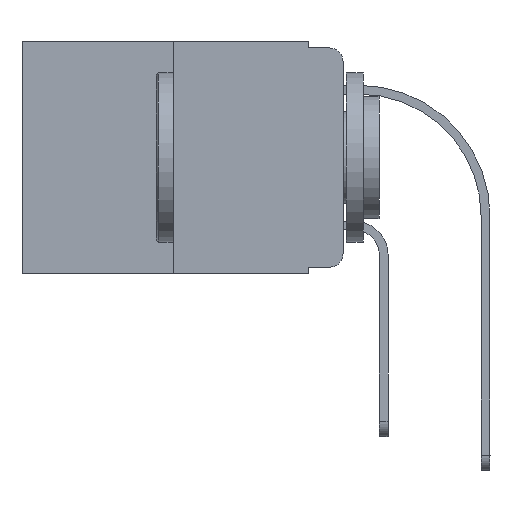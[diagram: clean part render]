
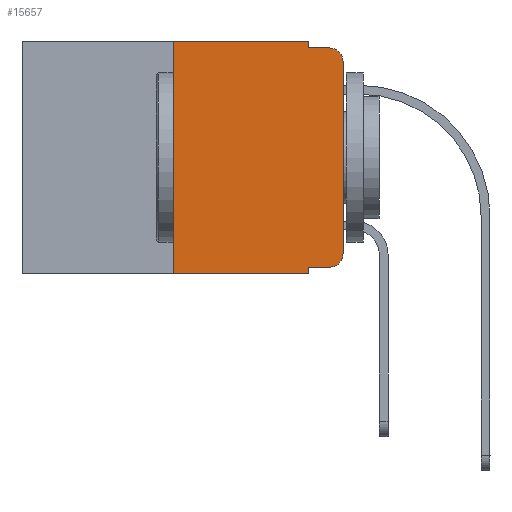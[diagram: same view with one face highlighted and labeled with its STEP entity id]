
A CAD part, left-side view. The second image highlights one B-rep face of the part: STEP entity #15657.
In plain terms, the highlighted planar face has unit normal (-1, 0, 0).
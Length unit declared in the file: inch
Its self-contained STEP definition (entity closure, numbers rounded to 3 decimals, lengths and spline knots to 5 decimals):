
#469 = VECTOR ( 'NONE', #5911, 39.37008 ) ;
#667 = EDGE_CURVE ( 'NONE', #11719, #19846, #1559, .T. ) ;
#905 = AXIS2_PLACEMENT_3D ( 'NONE', #5419, #11566, #17721 ) ;
#948 = CARTESIAN_POINT ( 'NONE',  ( 0., 0.051, 0. ) ) ;
#1408 = LINE ( 'NONE', #10692, #19639 ) ;
#1559 = LINE ( 'NONE', #7807, #7403 ) ;
#1925 = VERTEX_POINT ( 'NONE', #3932 ) ;
#1961 = LINE ( 'NONE', #11256, #14362 ) ;
#2019 = ORIENTED_EDGE ( 'NONE', *, *, #12223, .T. ) ;
#2073 = DIRECTION ( 'NONE',  ( 1., 0., 0. ) ) ;
#2264 = CARTESIAN_POINT ( 'NONE',  ( 0., 0.25, 0. ) ) ;
#2600 = CARTESIAN_POINT ( 'NONE',  ( 0., 0.051, 0. ) ) ;
#3450 = ORIENTED_EDGE ( 'NONE', *, *, #13535, .T. ) ;
#3794 = DIRECTION ( 'NONE',  ( 0., 0., -1. ) ) ;
#3808 = VERTEX_POINT ( 'NONE', #15187 ) ;
#3932 = CARTESIAN_POINT ( 'NONE',  ( 0., 0.051, -0.01 ) ) ;
#4041 = EDGE_CURVE ( 'NONE', #3808, #6773, #12874, .T. ) ;
#4103 = ORIENTED_EDGE ( 'NONE', *, *, #8879, .T. ) ;
#4409 = ORIENTED_EDGE ( 'NONE', *, *, #13688, .F. ) ;
#4512 = VECTOR ( 'NONE', #7450, 39.37008 ) ;
#4573 = ORIENTED_EDGE ( 'NONE', *, *, #9491, .F. ) ;
#4857 = CARTESIAN_POINT ( 'NONE',  ( 0., 0.02, -0.333 ) ) ;
#5004 = DIRECTION ( 'NONE',  ( 0., 0., 1. ) ) ;
#5223 = CARTESIAN_POINT ( 'NONE',  ( 0., 0.473, 0. ) ) ;
#5419 = CARTESIAN_POINT ( 'NONE',  ( 0., 0.02, -0.313 ) ) ;
#5911 = DIRECTION ( 'NONE',  ( 0., 0., -1. ) ) ;
#6040 = CARTESIAN_POINT ( 'NONE',  ( 0., 0.25, 0. ) ) ;
#6282 = CARTESIAN_POINT ( 'NONE',  ( 0., 0.25, -0.343 ) ) ;
#6498 = ORIENTED_EDGE ( 'NONE', *, *, #667, .T. ) ;
#6768 = CARTESIAN_POINT ( 'NONE',  ( 0., 0.02, -0.03 ) ) ;
#6773 = VERTEX_POINT ( 'NONE', #13117 ) ;
#7403 = VECTOR ( 'NONE', #5004, 39.37008 ) ;
#7450 = DIRECTION ( 'NONE',  ( 0., 0., 1. ) ) ;
#7468 = VERTEX_POINT ( 'NONE', #2264 ) ;
#7784 = DIRECTION ( 'NONE',  ( 0., -1., 0. ) ) ;
#7807 = CARTESIAN_POINT ( 'NONE',  ( 0., 0., 0. ) ) ;
#8496 = AXIS2_PLACEMENT_3D ( 'NONE', #5223, #2073, #19440 ) ;
#8706 = ORIENTED_EDGE ( 'NONE', *, *, #9300, .F. ) ;
#8800 = CARTESIAN_POINT ( 'NONE',  ( 0., 0.473, -0.343 ) ) ;
#8879 = EDGE_CURVE ( 'NONE', #16035, #6773, #17708, .T. ) ;
#8888 = ORIENTED_EDGE ( 'NONE', *, *, #12929, .T. ) ;
#9050 = EDGE_CURVE ( 'NONE', #1925, #17843, #10516, .T. ) ;
#9300 = EDGE_CURVE ( 'NONE', #10753, #1925, #14895, .T. ) ;
#9491 = EDGE_CURVE ( 'NONE', #7468, #10753, #1961, .T. ) ;
#9594 = CIRCLE ( 'NONE', #905, 0.02 ) ;
#10187 = DIRECTION ( 'NONE',  ( 0., 0., -1. ) ) ;
#10516 = LINE ( 'NONE', #12144, #13065 ) ;
#10692 = CARTESIAN_POINT ( 'NONE',  ( 0., 0.051, -0.333 ) ) ;
#10744 = CARTESIAN_POINT ( 'NONE',  ( 0., 0.051, 0. ) ) ;
#10753 = VERTEX_POINT ( 'NONE', #10744 ) ;
#11040 = CARTESIAN_POINT ( 'NONE',  ( 0., 0., -0.03 ) ) ;
#11256 = CARTESIAN_POINT ( 'NONE',  ( 0., 0.473, 0. ) ) ;
#11467 = FACE_OUTER_BOUND ( 'NONE', #16410, .T. ) ;
#11566 = DIRECTION ( 'NONE',  ( -1., 0., 0. ) ) ;
#11571 = PLANE ( 'NONE',  #8496 ) ;
#11614 = DIRECTION ( 'NONE',  ( -1., 0., 0. ) ) ;
#11654 = DIRECTION ( 'NONE',  ( 0., -1., 0. ) ) ;
#11719 = VERTEX_POINT ( 'NONE', #13028 ) ;
#12144 = CARTESIAN_POINT ( 'NONE',  ( 0., 0.051, -0.01 ) ) ;
#12223 = EDGE_CURVE ( 'NONE', #19117, #11719, #9594, .T. ) ;
#12521 = DIRECTION ( 'NONE',  ( 0., -1., 0. ) ) ;
#12546 = AXIS2_PLACEMENT_3D ( 'NONE', #6768, #11614, #10187 ) ;
#12874 = LINE ( 'NONE', #948, #18401 ) ;
#12929 = EDGE_CURVE ( 'NONE', #3808, #19117, #1408, .T. ) ;
#13028 = CARTESIAN_POINT ( 'NONE',  ( 0., 0., -0.313 ) ) ;
#13065 = VECTOR ( 'NONE', #7784, 39.37008 ) ;
#13080 = DIRECTION ( 'NONE',  ( 0., -1., 0. ) ) ;
#13117 = CARTESIAN_POINT ( 'NONE',  ( 0., 0.051, -0.343 ) ) ;
#13535 = EDGE_CURVE ( 'NONE', #19846, #17843, #18026, .T. ) ;
#13688 = EDGE_CURVE ( 'NONE', #16035, #7468, #14925, .T. ) ;
#13900 = ORIENTED_EDGE ( 'NONE', *, *, #9050, .F. ) ;
#14362 = VECTOR ( 'NONE', #13080, 39.37008 ) ;
#14407 = VECTOR ( 'NONE', #11654, 39.37008 ) ;
#14895 = LINE ( 'NONE', #2600, #469 ) ;
#14925 = LINE ( 'NONE', #6040, #4512 ) ;
#15187 = CARTESIAN_POINT ( 'NONE',  ( 0., 0.051, -0.333 ) ) ;
#15657 = ADVANCED_FACE ( 'NONE', ( #11467 ), #11571, .F. ) ;
#16035 = VERTEX_POINT ( 'NONE', #6282 ) ;
#16152 = ORIENTED_EDGE ( 'NONE', *, *, #4041, .F. ) ;
#16410 = EDGE_LOOP ( 'NONE', ( #6498, #3450, #13900, #8706, #4573, #4409, #4103, #16152, #8888, #2019 ) ) ;
#17708 = LINE ( 'NONE', #8800, #14407 ) ;
#17721 = DIRECTION ( 'NONE',  ( 0., 0., -1. ) ) ;
#17843 = VERTEX_POINT ( 'NONE', #17849 ) ;
#17849 = CARTESIAN_POINT ( 'NONE',  ( 0., 0.02, -0.01 ) ) ;
#18026 = CIRCLE ( 'NONE', #12546, 0.02 ) ;
#18401 = VECTOR ( 'NONE', #3794, 39.37008 ) ;
#19117 = VERTEX_POINT ( 'NONE', #4857 ) ;
#19440 = DIRECTION ( 'NONE',  ( 0., 0., -1. ) ) ;
#19639 = VECTOR ( 'NONE', #12521, 39.37008 ) ;
#19846 = VERTEX_POINT ( 'NONE', #11040 ) ;
